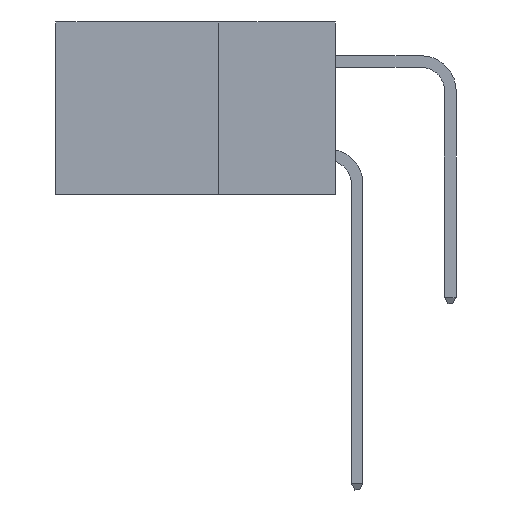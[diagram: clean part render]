
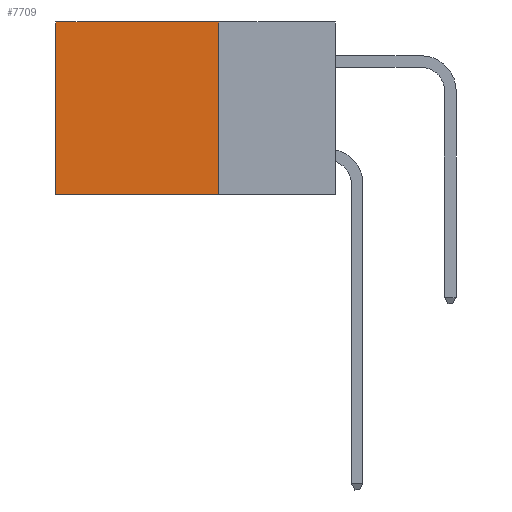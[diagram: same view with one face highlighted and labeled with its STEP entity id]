
A CAD part, left-side view. The second image highlights one B-rep face of the part: STEP entity #7709.
In plain terms, the highlighted planar face has unit normal (-1, 0, 0).
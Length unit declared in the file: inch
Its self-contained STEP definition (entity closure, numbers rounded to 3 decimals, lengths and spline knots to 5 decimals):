
#2691 = CARTESIAN_POINT ( 'NONE',  ( 0.2875, 0.25, -0.37 ) ) ;
#2902 = ORIENTED_EDGE ( 'NONE', *, *, #26870, .F. ) ;
#3657 = CARTESIAN_POINT ( 'NONE',  ( 0.2875, 0.25, 0. ) ) ;
#6347 = DIRECTION ( 'NONE',  ( 0., 1., 0. ) ) ;
#6840 = ORIENTED_EDGE ( 'NONE', *, *, #12495, .F. ) ;
#7150 = VERTEX_POINT ( 'NONE', #28519 ) ;
#7334 = DIRECTION ( 'NONE',  ( 0., 0., -1. ) ) ;
#7709 = ADVANCED_FACE ( 'NONE', ( #25791 ), #31397, .F. ) ;
#7710 = LINE ( 'NONE', #30781, #35084 ) ;
#8191 = LINE ( 'NONE', #24379, #46010 ) ;
#9324 = DIRECTION ( 'NONE',  ( 0., 1., 0. ) ) ;
#9694 = EDGE_CURVE ( 'NONE', #7150, #26416, #8191, .T. ) ;
#9970 = CARTESIAN_POINT ( 'NONE',  ( 0.2875, 0.25, 0. ) ) ;
#10128 = DIRECTION ( 'NONE',  ( 0., 0., -1. ) ) ;
#10230 = VECTOR ( 'NONE', #6347, 39.37008 ) ;
#10719 = LINE ( 'NONE', #2691, #10230 ) ;
#12495 = EDGE_CURVE ( 'NONE', #45145, #26416, #10719, .T. ) ;
#13193 = VERTEX_POINT ( 'NONE', #13631 ) ;
#13569 = DIRECTION ( 'NONE',  ( 1., 0., 0. ) ) ;
#13631 = CARTESIAN_POINT ( 'NONE',  ( 0.2875, 0.25, 0. ) ) ;
#15497 = CARTESIAN_POINT ( 'NONE',  ( 0.2875, 0.6, -0.37 ) ) ;
#16627 = LINE ( 'NONE', #3657, #23916 ) ;
#19360 = ORIENTED_EDGE ( 'NONE', *, *, #9694, .T. ) ;
#20288 = ORIENTED_EDGE ( 'NONE', *, *, #41671, .T. ) ;
#22813 = AXIS2_PLACEMENT_3D ( 'NONE', #9970, #13569, #38495 ) ;
#23916 = VECTOR ( 'NONE', #7334, 39.37008 ) ;
#24379 = CARTESIAN_POINT ( 'NONE',  ( 0.2875, 0.6, 0. ) ) ;
#25791 = FACE_OUTER_BOUND ( 'NONE', #37634, .T. ) ;
#26416 = VERTEX_POINT ( 'NONE', #15497 ) ;
#26870 = EDGE_CURVE ( 'NONE', #13193, #45145, #16627, .T. ) ;
#28519 = CARTESIAN_POINT ( 'NONE',  ( 0.2875, 0.6, 0. ) ) ;
#30781 = CARTESIAN_POINT ( 'NONE',  ( 0.2875, 0.25, 0. ) ) ;
#31397 = PLANE ( 'NONE',  #22813 ) ;
#35084 = VECTOR ( 'NONE', #9324, 39.37008 ) ;
#37634 = EDGE_LOOP ( 'NONE', ( #19360, #6840, #2902, #20288 ) ) ;
#38495 = DIRECTION ( 'NONE',  ( 0., 0., -1. ) ) ;
#41671 = EDGE_CURVE ( 'NONE', #13193, #7150, #7710, .T. ) ;
#45145 = VERTEX_POINT ( 'NONE', #45164 ) ;
#45164 = CARTESIAN_POINT ( 'NONE',  ( 0.2875, 0.25, -0.37 ) ) ;
#46010 = VECTOR ( 'NONE', #10128, 39.37008 ) ;
